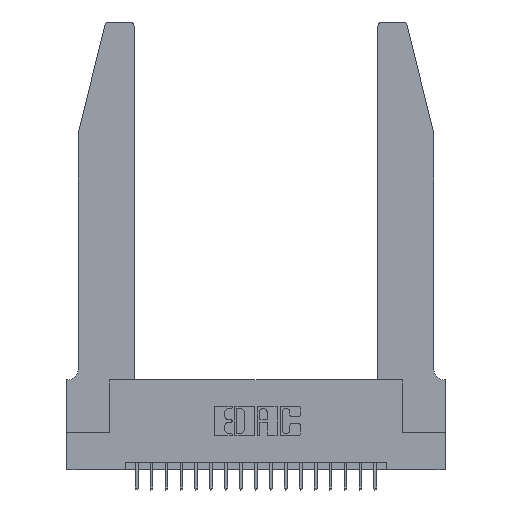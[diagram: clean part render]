
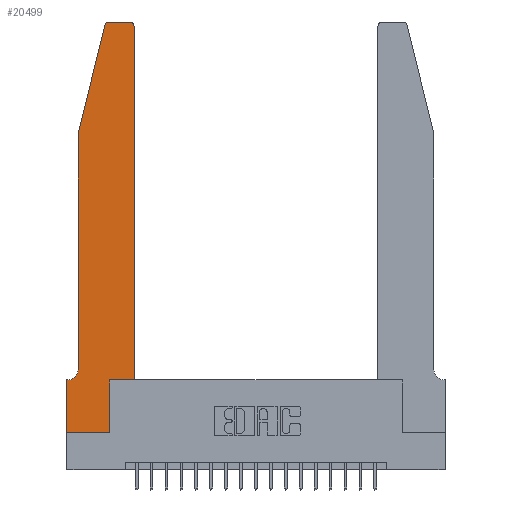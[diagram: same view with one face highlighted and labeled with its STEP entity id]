
A CAD part, top view. The second image highlights one B-rep face of the part: STEP entity #20499.
In plain terms, the highlighted planar face has unit normal (0, 0, 1).
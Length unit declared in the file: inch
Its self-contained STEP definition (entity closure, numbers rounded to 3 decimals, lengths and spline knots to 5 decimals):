
#4 = DIRECTION ( 'NONE',  ( 0., 0., 1. ) ) ;
#38 = EDGE_LOOP ( 'NONE', ( #5594, #14647, #12576, #1439, #3932, #17039, #10619, #13015, #4914, #13851, #7111, #2140 ) ) ;
#180 = EDGE_CURVE ( 'NONE', #12790, #19963, #5728, .T. ) ;
#777 = CARTESIAN_POINT ( 'NONE',  ( 0.0755, 2., 0.37 ) ) ;
#960 = VERTEX_POINT ( 'NONE', #5866 ) ;
#1071 = CARTESIAN_POINT ( 'NONE',  ( 0.2865, 0.35, 0.37 ) ) ;
#1173 = EDGE_CURVE ( 'NONE', #12667, #19211, #2712, .T. ) ;
#1439 = ORIENTED_EDGE ( 'NONE', *, *, #7001, .T. ) ;
#1604 = LINE ( 'NONE', #4568, #8794 ) ;
#2136 = DIRECTION ( 'NONE',  ( -1., 0., 0. ) ) ;
#2140 = ORIENTED_EDGE ( 'NONE', *, *, #15824, .T. ) ;
#2278 = AXIS2_PLACEMENT_3D ( 'NONE', #11377, #8893, #2136 ) ;
#2299 = DIRECTION ( 'NONE',  ( 0., -1., 0. ) ) ;
#2607 = VECTOR ( 'NONE', #11542, 39.37008 ) ;
#2698 = AXIS2_PLACEMENT_3D ( 'NONE', #4990, #10325, #15143 ) ;
#2712 = LINE ( 'NONE', #1071, #10051 ) ;
#3351 = VERTEX_POINT ( 'NONE', #9104 ) ;
#3486 = CARTESIAN_POINT ( 'NONE',  ( 0.25487, 2.72718, 0.37 ) ) ;
#3601 = DIRECTION ( 'NONE',  ( 1., 0., 0. ) ) ;
#3668 = VERTEX_POINT ( 'NONE', #9590 ) ;
#3678 = CARTESIAN_POINT ( 'NONE',  ( 0.0755, 0.35, 0.37 ) ) ;
#3718 = EDGE_CURVE ( 'NONE', #7327, #12667, #1604, .T. ) ;
#3932 = ORIENTED_EDGE ( 'NONE', *, *, #180, .T. ) ;
#4568 = CARTESIAN_POINT ( 'NONE',  ( 0., 0., 0.37 ) ) ;
#4792 = LINE ( 'NONE', #6519, #2607 ) ;
#4914 = ORIENTED_EDGE ( 'NONE', *, *, #1173, .T. ) ;
#4990 = CARTESIAN_POINT ( 'NONE',  ( 0.284, 2.72, 0.37 ) ) ;
#5181 = LINE ( 'NONE', #20031, #10112 ) ;
#5594 = ORIENTED_EDGE ( 'NONE', *, *, #11577, .T. ) ;
#5728 = CIRCLE ( 'NONE', #2278, 0.07 ) ;
#5797 = DIRECTION ( 'NONE',  ( 1., 0., 0. ) ) ;
#5866 = CARTESIAN_POINT ( 'NONE',  ( 0.284, 2.75, 0.37 ) ) ;
#6499 = EDGE_CURVE ( 'NONE', #3351, #7327, #13414, .T. ) ;
#6519 = CARTESIAN_POINT ( 'NONE',  ( 0.2605, 2.75, 0.37 ) ) ;
#6642 = EDGE_CURVE ( 'NONE', #16512, #3668, #15611, .T. ) ;
#6744 = LINE ( 'NONE', #13503, #20890 ) ;
#6992 = VECTOR ( 'NONE', #2299, 39.37008 ) ;
#6993 = VECTOR ( 'NONE', #9949, 39.37008 ) ;
#7001 = EDGE_CURVE ( 'NONE', #3668, #12790, #5181, .T. ) ;
#7111 = ORIENTED_EDGE ( 'NONE', *, *, #21198, .T. ) ;
#7190 = CARTESIAN_POINT ( 'NONE',  ( 0., 0., 0.37 ) ) ;
#7327 = VERTEX_POINT ( 'NONE', #14192 ) ;
#7907 = AXIS2_PLACEMENT_3D ( 'NONE', #20771, #16065, #5797 ) ;
#8262 = DIRECTION ( 'NONE',  ( 1., 0., 0. ) ) ;
#8501 = CARTESIAN_POINT ( 'NONE',  ( 0., 0.35, 0.37 ) ) ;
#8527 = EDGE_CURVE ( 'NONE', #19963, #3351, #11624, .T. ) ;
#8794 = VECTOR ( 'NONE', #8262, 39.37008 ) ;
#8893 = DIRECTION ( 'NONE',  ( 0., 0., -1. ) ) ;
#9078 = CARTESIAN_POINT ( 'NONE',  ( 0.4505, 2.72, 0.37 ) ) ;
#9104 = CARTESIAN_POINT ( 'NONE',  ( 0., 0.35, 0.37 ) ) ;
#9590 = CARTESIAN_POINT ( 'NONE',  ( 0.0755, 2., 0.37 ) ) ;
#9838 = CARTESIAN_POINT ( 'NONE',  ( 0.4505, 0.35, 0.37 ) ) ;
#9949 = DIRECTION ( 'NONE',  ( 0., 1., 0. ) ) ;
#10003 = VERTEX_POINT ( 'NONE', #17089 ) ;
#10051 = VECTOR ( 'NONE', #12828, 39.37008 ) ;
#10088 = DIRECTION ( 'NONE',  ( 0., -1., 0. ) ) ;
#10112 = VECTOR ( 'NONE', #10088, 39.37008 ) ;
#10325 = DIRECTION ( 'NONE',  ( 0., 0., 1. ) ) ;
#10564 = VECTOR ( 'NONE', #20157, 39.37008 ) ;
#10619 = ORIENTED_EDGE ( 'NONE', *, *, #6499, .T. ) ;
#10906 = VERTEX_POINT ( 'NONE', #17152 ) ;
#11377 = CARTESIAN_POINT ( 'NONE',  ( 0.0055, 0.42, 0.37 ) ) ;
#11542 = DIRECTION ( 'NONE',  ( -1., 0., 0. ) ) ;
#11577 = EDGE_CURVE ( 'NONE', #10003, #960, #4792, .T. ) ;
#11624 = LINE ( 'NONE', #3678, #10564 ) ;
#11872 = PLANE ( 'NONE',  #19518 ) ;
#12088 = CIRCLE ( 'NONE', #2698, 0.03 ) ;
#12451 = CARTESIAN_POINT ( 'NONE',  ( 0.2865, 0., 0.37 ) ) ;
#12576 = ORIENTED_EDGE ( 'NONE', *, *, #6642, .T. ) ;
#12667 = VERTEX_POINT ( 'NONE', #12451 ) ;
#12790 = VERTEX_POINT ( 'NONE', #19442 ) ;
#12828 = DIRECTION ( 'NONE',  ( 0., 1., 0. ) ) ;
#13015 = ORIENTED_EDGE ( 'NONE', *, *, #3718, .T. ) ;
#13172 = DIRECTION ( 'NONE',  ( 1., 0., 0. ) ) ;
#13414 = LINE ( 'NONE', #7190, #6992 ) ;
#13503 = CARTESIAN_POINT ( 'NONE',  ( 0.4505, 0.35, 0.37 ) ) ;
#13773 = CARTESIAN_POINT ( 'NONE',  ( 0.2865, 0.35, 0.37 ) ) ;
#13851 = ORIENTED_EDGE ( 'NONE', *, *, #17518, .T. ) ;
#14192 = CARTESIAN_POINT ( 'NONE',  ( 0., 0., 0.37 ) ) ;
#14647 = ORIENTED_EDGE ( 'NONE', *, *, #15345, .T. ) ;
#15143 = DIRECTION ( 'NONE',  ( 1., 0., 0. ) ) ;
#15345 = EDGE_CURVE ( 'NONE', #960, #16512, #12088, .T. ) ;
#15611 = LINE ( 'NONE', #777, #19548 ) ;
#15824 = EDGE_CURVE ( 'NONE', #17340, #10003, #15953, .T. ) ;
#15953 = CIRCLE ( 'NONE', #7907, 0.03 ) ;
#16065 = DIRECTION ( 'NONE',  ( 0., 0., 1. ) ) ;
#16512 = VERTEX_POINT ( 'NONE', #3486 ) ;
#17039 = ORIENTED_EDGE ( 'NONE', *, *, #8527, .T. ) ;
#17089 = CARTESIAN_POINT ( 'NONE',  ( 0.4205, 2.75, 0.37 ) ) ;
#17152 = CARTESIAN_POINT ( 'NONE',  ( 0.4505, 0.35, 0.37 ) ) ;
#17340 = VERTEX_POINT ( 'NONE', #9078 ) ;
#17518 = EDGE_CURVE ( 'NONE', #19211, #10906, #6744, .T. ) ;
#17653 = DIRECTION ( 'NONE',  ( -0.239, -0.971, 0. ) ) ;
#18003 = CARTESIAN_POINT ( 'NONE',  ( 0.0055, 0.35, 0.37 ) ) ;
#18541 = FACE_OUTER_BOUND ( 'NONE', #38, .T. ) ;
#19211 = VERTEX_POINT ( 'NONE', #13773 ) ;
#19442 = CARTESIAN_POINT ( 'NONE',  ( 0.0755, 0.42, 0.37 ) ) ;
#19518 = AXIS2_PLACEMENT_3D ( 'NONE', #8501, #4, #13172 ) ;
#19548 = VECTOR ( 'NONE', #17653, 39.37008 ) ;
#19963 = VERTEX_POINT ( 'NONE', #18003 ) ;
#20031 = CARTESIAN_POINT ( 'NONE',  ( 0.0755, 2., 0.37 ) ) ;
#20157 = DIRECTION ( 'NONE',  ( -1., 0., 0. ) ) ;
#20499 = ADVANCED_FACE ( 'NONE', ( #18541 ), #11872, .T. ) ;
#20771 = CARTESIAN_POINT ( 'NONE',  ( 0.4205, 2.72, 0.37 ) ) ;
#20890 = VECTOR ( 'NONE', #3601, 39.37008 ) ;
#21186 = LINE ( 'NONE', #9838, #6993 ) ;
#21198 = EDGE_CURVE ( 'NONE', #10906, #17340, #21186, .T. ) ;
